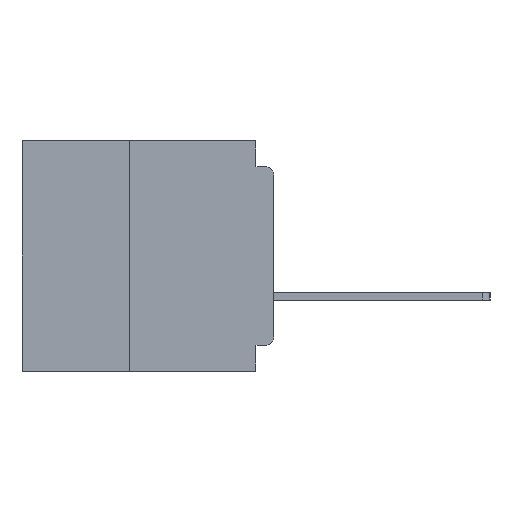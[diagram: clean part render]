
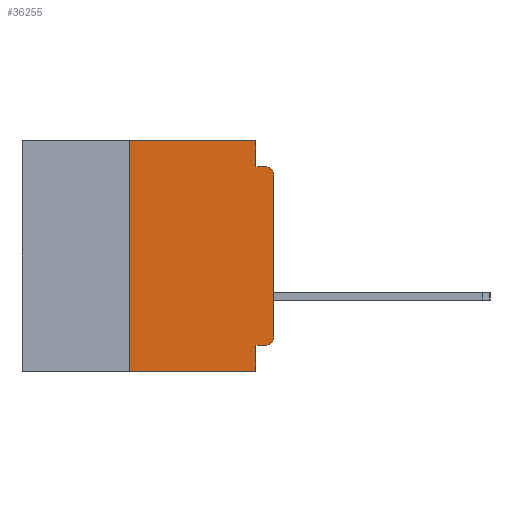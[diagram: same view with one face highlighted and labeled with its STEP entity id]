
A CAD part, left-side view. The second image highlights one B-rep face of the part: STEP entity #36255.
In plain terms, the highlighted planar face has unit normal (-1, 0, 0).
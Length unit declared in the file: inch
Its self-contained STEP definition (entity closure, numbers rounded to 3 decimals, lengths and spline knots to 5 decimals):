
#1051 = DIRECTION ( 'NONE',  ( 0., 0., -1. ) ) ;
#1160 = DIRECTION ( 'NONE',  ( 0., 0., -1. ) ) ;
#1948 = CARTESIAN_POINT ( 'NONE',  ( 0., 0.031, -0.045 ) ) ;
#3207 = VECTOR ( 'NONE', #33704, 39.37008 ) ;
#4510 = CARTESIAN_POINT ( 'NONE',  ( 0., 0., -0.34 ) ) ;
#5122 = DIRECTION ( 'NONE',  ( 0., 0., -1. ) ) ;
#5879 = EDGE_CURVE ( 'NONE', #8426, #39887, #13223, .T. ) ;
#6977 = EDGE_CURVE ( 'NONE', #57745, #36429, #60016, .T. ) ;
#8426 = VERTEX_POINT ( 'NONE', #13128 ) ;
#10643 = LINE ( 'NONE', #29186, #59890 ) ;
#10734 = PLANE ( 'NONE',  #35467 ) ;
#11218 = VECTOR ( 'NONE', #18803, 39.37008 ) ;
#11661 = FACE_OUTER_BOUND ( 'NONE', #42531, .T. ) ;
#12193 = CARTESIAN_POINT ( 'NONE',  ( 0., 0.031, -0.355 ) ) ;
#12389 = CARTESIAN_POINT ( 'NONE',  ( 0., 0.015, -0.045 ) ) ;
#13096 = CARTESIAN_POINT ( 'NONE',  ( 0., 0.437, -0.4 ) ) ;
#13128 = CARTESIAN_POINT ( 'NONE',  ( 0., 0.25, -0.4 ) ) ;
#13223 = LINE ( 'NONE', #23507, #24648 ) ;
#13553 = EDGE_CURVE ( 'NONE', #50316, #24410, #10643, .T. ) ;
#17969 = DIRECTION ( 'NONE',  ( 0., -1., 0. ) ) ;
#18606 = DIRECTION ( 'NONE',  ( 0., 0., 1. ) ) ;
#18752 = EDGE_CURVE ( 'NONE', #57794, #50316, #50397, .T. ) ;
#18803 = DIRECTION ( 'NONE',  ( 0., 0., 1. ) ) ;
#18831 = CARTESIAN_POINT ( 'NONE',  ( 0., 0.031, 0. ) ) ;
#19900 = DIRECTION ( 'NONE',  ( 0., -1., 0. ) ) ;
#20110 = VECTOR ( 'NONE', #38246, 39.37008 ) ;
#20614 = CARTESIAN_POINT ( 'NONE',  ( 0., 0., -0.06 ) ) ;
#23507 = CARTESIAN_POINT ( 'NONE',  ( 0., 0.25, -0.4 ) ) ;
#23523 = CARTESIAN_POINT ( 'NONE',  ( 0., 0.015, -0.355 ) ) ;
#24071 = EDGE_CURVE ( 'NONE', #39887, #57794, #41572, .T. ) ;
#24410 = VERTEX_POINT ( 'NONE', #12389 ) ;
#24511 = CARTESIAN_POINT ( 'NONE',  ( 0., 0.031, 0. ) ) ;
#24648 = VECTOR ( 'NONE', #18606, 39.37008 ) ;
#25848 = EDGE_CURVE ( 'NONE', #36429, #42352, #59458, .T. ) ;
#28355 = CARTESIAN_POINT ( 'NONE',  ( 0., 0.015, -0.34 ) ) ;
#28662 = AXIS2_PLACEMENT_3D ( 'NONE', #58414, #30107, #1051 ) ;
#28966 = CARTESIAN_POINT ( 'NONE',  ( 0., 0.437, 0. ) ) ;
#29186 = CARTESIAN_POINT ( 'NONE',  ( 0., 0., -0.045 ) ) ;
#29187 = ORIENTED_EDGE ( 'NONE', *, *, #6977, .F. ) ;
#29366 = ORIENTED_EDGE ( 'NONE', *, *, #18752, .F. ) ;
#30107 = DIRECTION ( 'NONE',  ( -1., 0., 0. ) ) ;
#30214 = DIRECTION ( 'NONE',  ( 1., 0., 0. ) ) ;
#30977 = CARTESIAN_POINT ( 'NONE',  ( 0., 0.031, -0.4 ) ) ;
#32331 = CIRCLE ( 'NONE', #28662, 0.015 ) ;
#33137 = DIRECTION ( 'NONE',  ( 0., 0., -1. ) ) ;
#33520 = CARTESIAN_POINT ( 'NONE',  ( 0., 0.031, -0.4 ) ) ;
#33704 = DIRECTION ( 'NONE',  ( 0., -1., 0. ) ) ;
#33915 = ORIENTED_EDGE ( 'NONE', *, *, #49832, .T. ) ;
#34424 = ORIENTED_EDGE ( 'NONE', *, *, #45447, .T. ) ;
#34887 = VECTOR ( 'NONE', #40095, 39.37008 ) ;
#34929 = LINE ( 'NONE', #13096, #58591 ) ;
#35467 = AXIS2_PLACEMENT_3D ( 'NONE', #58505, #30214, #1160 ) ;
#36255 = ADVANCED_FACE ( 'NONE', ( #11661 ), #10734, .F. ) ;
#36429 = VERTEX_POINT ( 'NONE', #12193 ) ;
#38092 = ORIENTED_EDGE ( 'NONE', *, *, #24071, .F. ) ;
#38246 = DIRECTION ( 'NONE',  ( 0., 0., -1. ) ) ;
#39434 = ORIENTED_EDGE ( 'NONE', *, *, #47178, .T. ) ;
#39887 = VERTEX_POINT ( 'NONE', #61219 ) ;
#40095 = DIRECTION ( 'NONE',  ( 0., 1., 0. ) ) ;
#40578 = AXIS2_PLACEMENT_3D ( 'NONE', #28355, #61414, #33137 ) ;
#41572 = LINE ( 'NONE', #28966, #3207 ) ;
#42011 = ORIENTED_EDGE ( 'NONE', *, *, #13553, .F. ) ;
#42150 = VERTEX_POINT ( 'NONE', #4510 ) ;
#42352 = VERTEX_POINT ( 'NONE', #30977 ) ;
#42531 = EDGE_LOOP ( 'NONE', ( #53403, #34424, #42011, #29366, #38092, #47493, #33915, #43142, #29187, #39434 ) ) ;
#43142 = ORIENTED_EDGE ( 'NONE', *, *, #25848, .F. ) ;
#45447 = EDGE_CURVE ( 'NONE', #46802, #24410, #32331, .T. ) ;
#45993 = EDGE_CURVE ( 'NONE', #42150, #46802, #61902, .T. ) ;
#46802 = VERTEX_POINT ( 'NONE', #20614 ) ;
#47178 = EDGE_CURVE ( 'NONE', #57745, #42150, #53620, .T. ) ;
#47493 = ORIENTED_EDGE ( 'NONE', *, *, #5879, .F. ) ;
#48954 = VECTOR ( 'NONE', #5122, 39.37008 ) ;
#49638 = CARTESIAN_POINT ( 'NONE',  ( 0., 0., -0.355 ) ) ;
#49832 = EDGE_CURVE ( 'NONE', #8426, #42352, #34929, .T. ) ;
#50316 = VERTEX_POINT ( 'NONE', #1948 ) ;
#50397 = LINE ( 'NONE', #24511, #48954 ) ;
#52038 = CARTESIAN_POINT ( 'NONE',  ( 0., 0., 0. ) ) ;
#53403 = ORIENTED_EDGE ( 'NONE', *, *, #45993, .T. ) ;
#53620 = CIRCLE ( 'NONE', #40578, 0.015 ) ;
#57745 = VERTEX_POINT ( 'NONE', #23523 ) ;
#57794 = VERTEX_POINT ( 'NONE', #18831 ) ;
#58414 = CARTESIAN_POINT ( 'NONE',  ( 0., 0.015, -0.06 ) ) ;
#58505 = CARTESIAN_POINT ( 'NONE',  ( 0., 0.437, 0. ) ) ;
#58591 = VECTOR ( 'NONE', #17969, 39.37008 ) ;
#59458 = LINE ( 'NONE', #33520, #20110 ) ;
#59890 = VECTOR ( 'NONE', #19900, 39.37008 ) ;
#60016 = LINE ( 'NONE', #49638, #34887 ) ;
#61219 = CARTESIAN_POINT ( 'NONE',  ( 0., 0.25, 0. ) ) ;
#61414 = DIRECTION ( 'NONE',  ( -1., 0., 0. ) ) ;
#61902 = LINE ( 'NONE', #52038, #11218 ) ;
